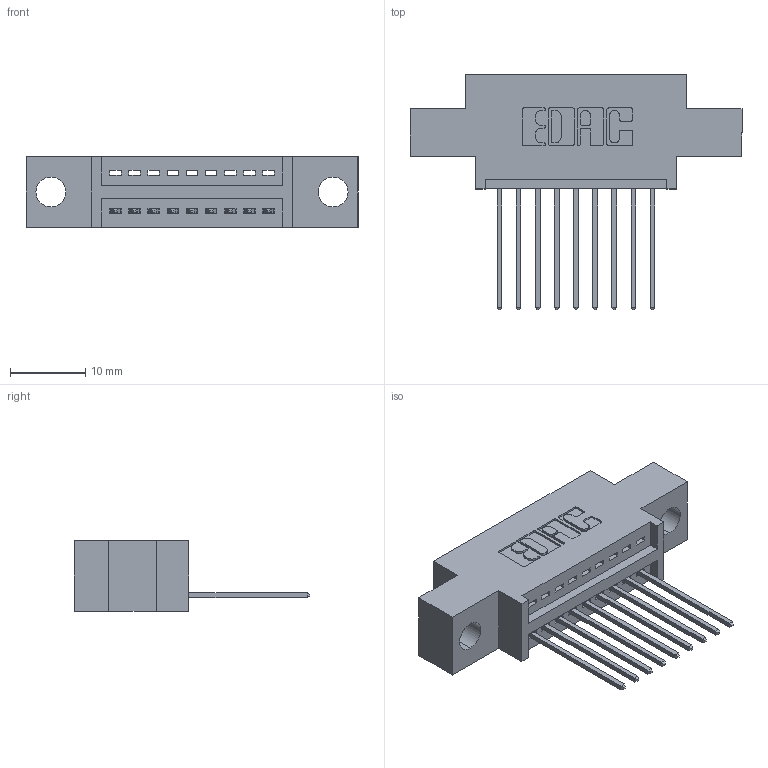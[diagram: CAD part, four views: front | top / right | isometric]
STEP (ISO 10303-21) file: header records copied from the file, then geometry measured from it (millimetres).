
FILE_DESCRIPTION (( 'STEP AP203' ), '1' );
FILE_NAME ('345-009-542-604.STEP', '2021-05-26T14:04:50', ( '' ), ( '' ), 'SwSTEP 2.0', 'SolidWorks 2020', '' );
FILE_SCHEMA (( 'CONFIG_CONTROL_DESIGN' ));
Length unit declared in the file: inch
Products named in the file (3): 345-009-542-604; 345-292-001_345-293-142; 345 Part_0.170 Offset - 0.156 Dia-TI
Assembly tree (10 placements, depth 2):
  345-009-542-604
    345 Part_0.170 Offset - 0.156 Dia-TI
    345-292-001_345-293-142  x9
Bounding box: 44.07 x 31.29 x 9.4 mm (x, y, z)
Volume: 3716.1 mm3; surface area: 4585.5 mm2
Topology: 10 solids, 10 shells, 666 faces, 1973 edges, 1302 vertices
Faces by surface type: plane 458, cylinder 208
Entity records: 11785 total; most frequent: CARTESIAN_POINT 2053, ORIENTED_EDGE 1994, DIRECTION 1839, EDGE_CURVE 997, VECTOR 829, LINE 829, VERTEX_POINT 662, AXIS2_PLACEMENT_3D 505
